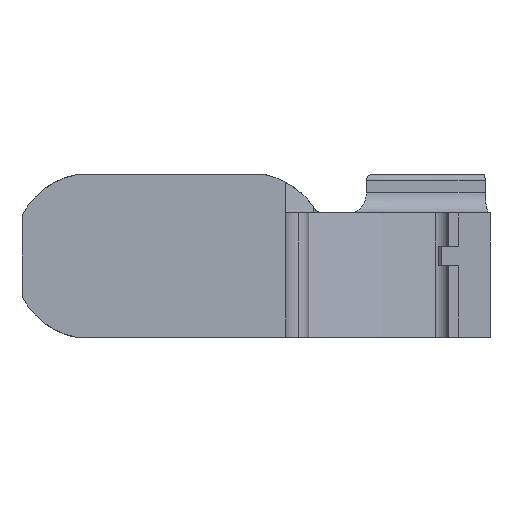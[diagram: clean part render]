
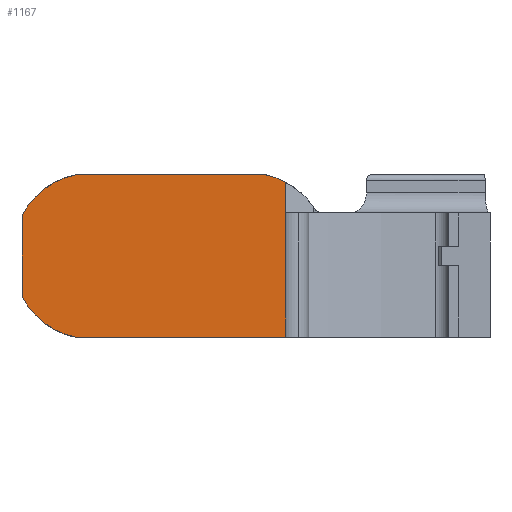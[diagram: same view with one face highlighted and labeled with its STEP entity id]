
A CAD part, front view. The second image highlights one B-rep face of the part: STEP entity #1167.
In plain terms, the highlighted planar face has unit normal (0, -1, 0).
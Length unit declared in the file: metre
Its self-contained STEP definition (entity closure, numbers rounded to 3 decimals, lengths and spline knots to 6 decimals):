
#103=CIRCLE('',#1299,0.005934);
#104=CIRCLE('',#1300,0.005934);
#105=CIRCLE('',#1301,0.005934);
#150=FACE_OUTER_BOUND('',#211,.T.);
#211=EDGE_LOOP('',(#994,#995,#996,#997,#998,#999,#1000));
#245=LINE('',#1734,#358);
#263=LINE('',#1794,#376);
#324=LINE('',#1972,#437);
#325=LINE('',#1975,#438);
#358=VECTOR('',#1379,0.014606);
#376=VECTOR('',#1431,0.016179);
#437=VECTOR('',#1602,0.006173);
#438=VECTOR('',#1605,0.011874);
#484=VERTEX_POINT('',#1731);
#485=VERTEX_POINT('',#1733);
#509=VERTEX_POINT('',#1791);
#510=VERTEX_POINT('',#1793);
#557=VERTEX_POINT('',#1969);
#558=VERTEX_POINT('',#1971);
#559=VERTEX_POINT('',#1974);
#601=EDGE_CURVE('',#484,#485,#245,.T.);
#631=EDGE_CURVE('',#510,#509,#263,.T.);
#714=EDGE_CURVE('',#484,#557,#103,.F.);
#715=EDGE_CURVE('',#557,#558,#324,.T.);
#716=EDGE_CURVE('',#558,#510,#104,.F.);
#717=EDGE_CURVE('',#559,#509,#325,.T.);
#718=EDGE_CURVE('',#485,#559,#105,.T.);
#994=ORIENTED_EDGE('',*,*,#601,.F.);
#995=ORIENTED_EDGE('',*,*,#714,.T.);
#996=ORIENTED_EDGE('',*,*,#715,.T.);
#997=ORIENTED_EDGE('',*,*,#716,.T.);
#998=ORIENTED_EDGE('',*,*,#631,.T.);
#999=ORIENTED_EDGE('',*,*,#717,.F.);
#1000=ORIENTED_EDGE('',*,*,#718,.F.);
#1117=PLANE('',#1298);
#1167=ADVANCED_FACE('',(#150),#1117,.F.);
#1298=AXIS2_PLACEMENT_3D('',#1968,#1598,#1599);
#1299=AXIS2_PLACEMENT_3D('',#1970,#1600,#1601);
#1300=AXIS2_PLACEMENT_3D('',#1973,#1603,#1604);
#1301=AXIS2_PLACEMENT_3D('',#1976,#1606,#1607);
#1379=DIRECTION('',(1.,0.,0.));
#1431=DIRECTION('',(1.,0.,0.));
#1598=DIRECTION('center_axis',(0.,1.,0.));
#1599=DIRECTION('ref_axis',(-1.,0.,0.));
#1600=DIRECTION('center_axis',(0.,1.,0.));
#1601=DIRECTION('ref_axis',(-1.,0.,0.));
#1602=DIRECTION('',(0.,0.,-1.));
#1603=DIRECTION('center_axis',(0.,1.,0.));
#1604=DIRECTION('ref_axis',(-1.,0.,0.));
#1605=DIRECTION('',(0.,0.,-1.));
#1606=DIRECTION('center_axis',(0.,1.,0.));
#1607=DIRECTION('ref_axis',(-1.,0.,0.));
#1731=CARTESIAN_POINT('',(-0.00605,-0.009525,0.00562));
#1733=CARTESIAN_POINT('',(0.008555,-0.009525,0.00562));
#1734=CARTESIAN_POINT('',(-0.00605,-0.009525,0.00562));
#1791=CARTESIAN_POINT('',(0.010128,-0.009525,-0.006826));
#1793=CARTESIAN_POINT('',(-0.00605,-0.009525,-0.006826));
#1794=CARTESIAN_POINT('',(-0.00605,-0.009525,-0.006826));
#1968=CARTESIAN_POINT('Origin',(-0.000603,-0.009525,0.00562));
#1969=CARTESIAN_POINT('',(-0.010128,-0.009525,0.002483));
#1970=CARTESIAN_POINT('Origin',(-0.004829,-0.009525,-0.000187));
#1971=CARTESIAN_POINT('',(-0.010128,-0.009525,-0.00369));
#1972=CARTESIAN_POINT('',(-0.010128,-0.009525,0.002483));
#1973=CARTESIAN_POINT('Origin',(-0.004829,-0.009525,-0.001019));
#1974=CARTESIAN_POINT('',(0.010128,-0.009525,0.005048));
#1975=CARTESIAN_POINT('',(0.010128,-0.009525,0.005048));
#1976=CARTESIAN_POINT('Origin',(0.007334,-0.009525,-0.000187));
